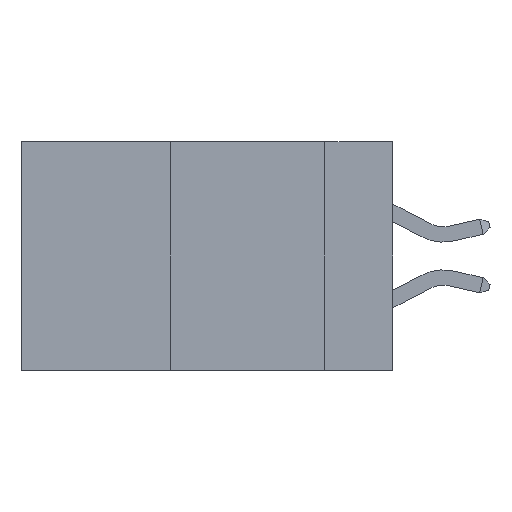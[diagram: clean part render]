
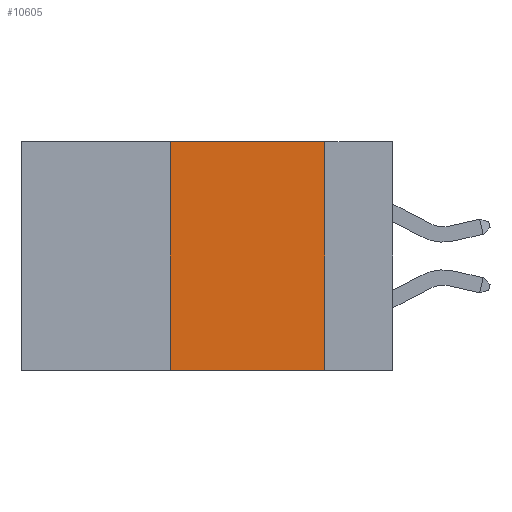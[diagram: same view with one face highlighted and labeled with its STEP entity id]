
A CAD part, left-side view. The second image highlights one B-rep face of the part: STEP entity #10605.
In plain terms, the highlighted planar face has unit normal (-1, 0, 0).
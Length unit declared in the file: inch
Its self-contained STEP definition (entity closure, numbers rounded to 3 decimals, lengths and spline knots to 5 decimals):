
#325 = CARTESIAN_POINT ( 'NONE',  ( 0., 0.36, -0.37 ) ) ;
#777 = ORIENTED_EDGE ( 'NONE', *, *, #3710, .F. ) ;
#1479 = DIRECTION ( 'NONE',  ( 1., 0., 0. ) ) ;
#3050 = VERTEX_POINT ( 'NONE', #9551 ) ;
#3052 = LINE ( 'NONE', #11908, #21143 ) ;
#3062 = CARTESIAN_POINT ( 'NONE',  ( 0., 0.6, 0. ) ) ;
#3710 = EDGE_CURVE ( 'NONE', #3050, #6074, #3959, .T. ) ;
#3959 = LINE ( 'NONE', #3062, #20928 ) ;
#5055 = CARTESIAN_POINT ( 'NONE',  ( 0., 0.6, 0. ) ) ;
#5206 = EDGE_CURVE ( 'NONE', #9947, #12434, #3052, .T. ) ;
#5331 = CARTESIAN_POINT ( 'NONE',  ( 0., 0.36, 0. ) ) ;
#5537 = DIRECTION ( 'NONE',  ( 0., 0., -1. ) ) ;
#6074 = VERTEX_POINT ( 'NONE', #15213 ) ;
#7236 = LINE ( 'NONE', #7526, #12900 ) ;
#7239 = ORIENTED_EDGE ( 'NONE', *, *, #8098, .F. ) ;
#7526 = CARTESIAN_POINT ( 'NONE',  ( 0., 0.11, 0. ) ) ;
#7529 = ORIENTED_EDGE ( 'NONE', *, *, #5206, .T. ) ;
#7827 = VECTOR ( 'NONE', #10478, 39.37008 ) ;
#8098 = EDGE_CURVE ( 'NONE', #9947, #3050, #17965, .T. ) ;
#8236 = EDGE_CURVE ( 'NONE', #6074, #12434, #7236, .T. ) ;
#9551 = CARTESIAN_POINT ( 'NONE',  ( 0., 0.36, 0. ) ) ;
#9562 = CARTESIAN_POINT ( 'NONE',  ( 0., 0.11, -0.37 ) ) ;
#9947 = VERTEX_POINT ( 'NONE', #325 ) ;
#10036 = DIRECTION ( 'NONE',  ( 0., -1., 0. ) ) ;
#10478 = DIRECTION ( 'NONE',  ( 0., 0., 1. ) ) ;
#10567 = FACE_OUTER_BOUND ( 'NONE', #19448, .T. ) ;
#10605 = ADVANCED_FACE ( 'NONE', ( #10567 ), #18774, .F. ) ;
#11908 = CARTESIAN_POINT ( 'NONE',  ( 0., 0.6, -0.37 ) ) ;
#12434 = VERTEX_POINT ( 'NONE', #9562 ) ;
#12900 = VECTOR ( 'NONE', #5537, 39.37008 ) ;
#13379 = DIRECTION ( 'NONE',  ( 0., -1., 0. ) ) ;
#15213 = CARTESIAN_POINT ( 'NONE',  ( 0., 0.11, 0. ) ) ;
#15513 = AXIS2_PLACEMENT_3D ( 'NONE', #5055, #1479, #21708 ) ;
#17965 = LINE ( 'NONE', #5331, #7827 ) ;
#18774 = PLANE ( 'NONE',  #15513 ) ;
#19448 = EDGE_LOOP ( 'NONE', ( #20153, #777, #7239, #7529 ) ) ;
#20153 = ORIENTED_EDGE ( 'NONE', *, *, #8236, .F. ) ;
#20928 = VECTOR ( 'NONE', #10036, 39.37008 ) ;
#21143 = VECTOR ( 'NONE', #13379, 39.37008 ) ;
#21708 = DIRECTION ( 'NONE',  ( 0., 0., -1. ) ) ;
